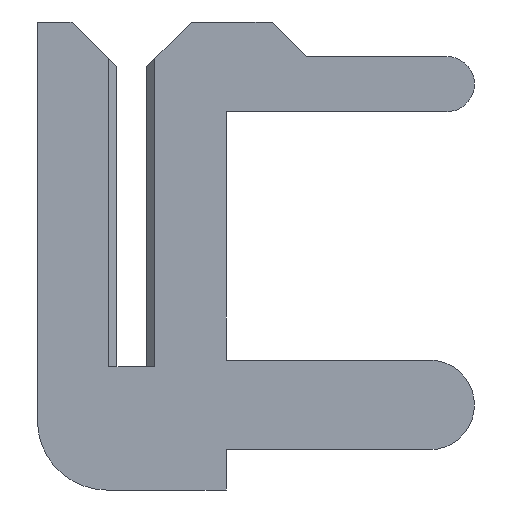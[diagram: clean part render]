
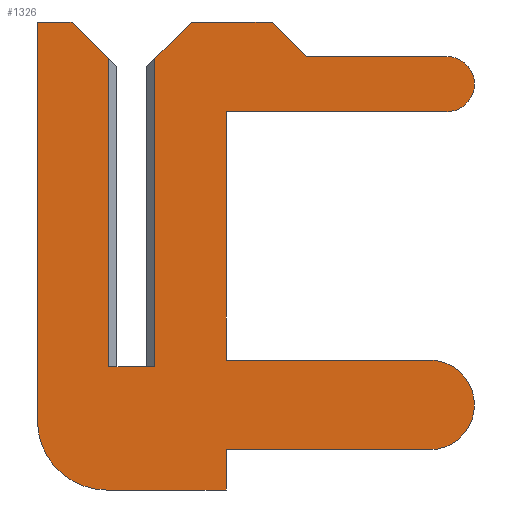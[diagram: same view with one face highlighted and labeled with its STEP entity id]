
A CAD part, left-side view. The second image highlights one B-rep face of the part: STEP entity #1326.
In plain terms, the highlighted planar face has unit normal (-1, 0, 0).
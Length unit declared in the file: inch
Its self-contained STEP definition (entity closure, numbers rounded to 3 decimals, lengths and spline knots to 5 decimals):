
#25 = VECTOR ( 'NONE', #924, 39.37008 ) ;
#30 = EDGE_CURVE ( 'NONE', #459, #676, #1230, .T. ) ;
#34 = CARTESIAN_POINT ( 'NONE',  ( -0.01, -0.041, -0.036 ) ) ;
#63 = DIRECTION ( 'NONE',  ( 0., 0., 1. ) ) ;
#75 = LINE ( 'NONE', #409, #1272 ) ;
#92 = CARTESIAN_POINT ( 'NONE',  ( -0.01, -0.041, -0.036 ) ) ;
#99 = ORIENTED_EDGE ( 'NONE', *, *, #148, .F. ) ;
#102 = CARTESIAN_POINT ( 'NONE',  ( -0.01, -0.1295, 0.003 ) ) ;
#108 = CIRCLE ( 'NONE', #139, 0.0195 ) ;
#113 = CARTESIAN_POINT ( 'NONE',  ( -0.01, -0.026, 0.15 ) ) ;
#116 = DIRECTION ( 'NONE',  ( 1., 0., 0. ) ) ;
#126 = VECTOR ( 'NONE', #713, 39.37008 ) ;
#127 = EDGE_CURVE ( 'NONE', #171, #828, #289, .T. ) ;
#139 = AXIS2_PLACEMENT_3D ( 'NONE', #839, #142, #849 ) ;
#142 = DIRECTION ( 'NONE',  ( 1., 0., 0. ) ) ;
#148 = EDGE_CURVE ( 'NONE', #936, #709, #663, .T. ) ;
#159 = VERTEX_POINT ( 'NONE', #92 ) ;
#171 = VERTEX_POINT ( 'NONE', #187 ) ;
#174 = DIRECTION ( 'NONE',  ( 1., 0., 0. ) ) ;
#179 = ORIENTED_EDGE ( 'NONE', *, *, #30, .F. ) ;
#186 = VECTOR ( 'NONE', #391, 39.37008 ) ;
#187 = CARTESIAN_POINT ( 'NONE',  ( -0.01, -0.041, -0.0535 ) ) ;
#191 = LINE ( 'NONE', #812, #1374 ) ;
#193 = ORIENTED_EDGE ( 'NONE', *, *, #1288, .F. ) ;
#198 = CARTESIAN_POINT ( 'NONE',  ( -0.01, -0.076, 0.135 ) ) ;
#202 = ORIENTED_EDGE ( 'NONE', *, *, #1087, .F. ) ;
#218 = ORIENTED_EDGE ( 'NONE', *, *, #1364, .F. ) ;
#219 = EDGE_CURVE ( 'NONE', #491, #324, #75, .T. ) ;
#234 = CARTESIAN_POINT ( 'NONE',  ( -0.01, -0.041, -0.0535 ) ) ;
#242 = DIRECTION ( 'NONE',  ( 0., 0., -1. ) ) ;
#253 = CARTESIAN_POINT ( 'NONE',  ( -0.01, -0.01, 0.134 ) ) ;
#268 = CARTESIAN_POINT ( 'NONE',  ( -0.01, -0.1295, 0.003 ) ) ;
#270 = VECTOR ( 'NONE', #474, 39.37008 ) ;
#289 = LINE ( 'NONE', #637, #1474 ) ;
#307 = ORIENTED_EDGE ( 'NONE', *, *, #879, .T. ) ;
#310 = LINE ( 'NONE', #342, #270 ) ;
#312 = VECTOR ( 'NONE', #1359, 39.37008 ) ;
#324 = VERTEX_POINT ( 'NONE', #526 ) ;
#336 = LINE ( 'NONE', #1060, #126 ) ;
#341 = EDGE_CURVE ( 'NONE', #1260, #595, #807, .T. ) ;
#342 = CARTESIAN_POINT ( 'NONE',  ( -0.01, 0.0065, 0. ) ) ;
#359 = DIRECTION ( 'NONE',  ( 0., 0., -1. ) ) ;
#373 = VECTOR ( 'NONE', #1048, 39.37008 ) ;
#380 = CARTESIAN_POINT ( 'NONE',  ( -0.01, 0.011, -0.0535 ) ) ;
#384 = CARTESIAN_POINT ( 'NONE',  ( -0.01, 0.011, -0.0235 ) ) ;
#391 = DIRECTION ( 'NONE',  ( 0., -1., 0. ) ) ;
#409 = CARTESIAN_POINT ( 'NONE',  ( -0.01, 0.0065, 0.1305 ) ) ;
#458 = CARTESIAN_POINT ( 'NONE',  ( -0.01, -0.137, 0.135 ) ) ;
#459 = VERTEX_POINT ( 'NONE', #1263 ) ;
#471 = ORIENTED_EDGE ( 'NONE', *, *, #1324, .F. ) ;
#473 = EDGE_CURVE ( 'NONE', #1168, #1331, #310, .T. ) ;
#474 = DIRECTION ( 'NONE',  ( 0., -1., 0. ) ) ;
#479 = CARTESIAN_POINT ( 'NONE',  ( -0.01, -0.0065, 0.1305 ) ) ;
#482 = CARTESIAN_POINT ( 'NONE',  ( -0.01, -0.026, 0.15 ) ) ;
#485 = LINE ( 'NONE', #234, #684 ) ;
#491 = VERTEX_POINT ( 'NONE', #926 ) ;
#496 = ORIENTED_EDGE ( 'NONE', *, *, #127, .F. ) ;
#505 = LINE ( 'NONE', #268, #186 ) ;
#517 = AXIS2_PLACEMENT_3D ( 'NONE', #384, #116, #825 ) ;
#526 = CARTESIAN_POINT ( 'NONE',  ( -0.01, 0.01, 0.134 ) ) ;
#531 = DIRECTION ( 'NONE',  ( 0., 1., 0. ) ) ;
#539 = VERTEX_POINT ( 'NONE', #458 ) ;
#562 = AXIS2_PLACEMENT_3D ( 'NONE', #1453, #174, #1429 ) ;
#595 = VERTEX_POINT ( 'NONE', #1037 ) ;
#597 = DIRECTION ( 'NONE',  ( 0., 0., 1. ) ) ;
#628 = LINE ( 'NONE', #1163, #870 ) ;
#637 = CARTESIAN_POINT ( 'NONE',  ( -0.01, 0.011, -0.0535 ) ) ;
#641 = VERTEX_POINT ( 'NONE', #102 ) ;
#647 = LINE ( 'NONE', #738, #702 ) ;
#660 = VECTOR ( 'NONE', #63, 39.37008 ) ;
#663 = LINE ( 'NONE', #1104, #312 ) ;
#676 = VERTEX_POINT ( 'NONE', #1307 ) ;
#684 = VECTOR ( 'NONE', #242, 39.37008 ) ;
#686 = EDGE_CURVE ( 'NONE', #828, #1260, #834, .T. ) ;
#687 = ORIENTED_EDGE ( 'NONE', *, *, #686, .F. ) ;
#698 = DIRECTION ( 'NONE',  ( 0., 1., 0. ) ) ;
#702 = VECTOR ( 'NONE', #880, 39.37008 ) ;
#707 = ORIENTED_EDGE ( 'NONE', *, *, #1242, .F. ) ;
#709 = VERTEX_POINT ( 'NONE', #1166 ) ;
#713 = DIRECTION ( 'NONE',  ( 0., 1., 0. ) ) ;
#715 = ORIENTED_EDGE ( 'NONE', *, *, #473, .F. ) ;
#732 = CARTESIAN_POINT ( 'NONE',  ( -0.01, -0.01, 0. ) ) ;
#738 = CARTESIAN_POINT ( 'NONE',  ( -0.01, -0.137, 0.135 ) ) ;
#748 = VERTEX_POINT ( 'NONE', #482 ) ;
#774 = ORIENTED_EDGE ( 'NONE', *, *, #1169, .F. ) ;
#780 = VECTOR ( 'NONE', #1391, 39.37008 ) ;
#785 = ORIENTED_EDGE ( 'NONE', *, *, #341, .F. ) ;
#807 = LINE ( 'NONE', #1325, #660 ) ;
#812 = CARTESIAN_POINT ( 'NONE',  ( -0.01, -0.01, 0.15 ) ) ;
#825 = DIRECTION ( 'NONE',  ( 0., 0., 1. ) ) ;
#828 = VERTEX_POINT ( 'NONE', #380 ) ;
#831 = VECTOR ( 'NONE', #698, 39.37008 ) ;
#834 = CIRCLE ( 'NONE', #517, 0.03 ) ;
#839 = CARTESIAN_POINT ( 'NONE',  ( -0.01, -0.1295, -0.0165 ) ) ;
#849 = DIRECTION ( 'NONE',  ( 0., 0., 1. ) ) ;
#870 = VECTOR ( 'NONE', #597, 39.37008 ) ;
#879 = EDGE_CURVE ( 'NONE', #1224, #1331, #191, .T. ) ;
#880 = DIRECTION ( 'NONE',  ( 0., -1., 0. ) ) ;
#885 = EDGE_LOOP ( 'NONE', ( #1437, #307, #715, #1167, #1149, #202, #785, #687, #496, #774, #1412, #193, #471, #99, #218, #1154, #1150, #179, #707 ) ) ;
#924 = DIRECTION ( 'NONE',  ( 0., -1., 0. ) ) ;
#926 = CARTESIAN_POINT ( 'NONE',  ( -0.01, 0.026, 0.15 ) ) ;
#931 = CARTESIAN_POINT ( 'NONE',  ( -0.01, 0.01, 0. ) ) ;
#936 = VERTEX_POINT ( 'NONE', #1202 ) ;
#944 = LINE ( 'NONE', #34, #831 ) ;
#958 = PLANE ( 'NONE',  #1228 ) ;
#992 = FACE_OUTER_BOUND ( 'NONE', #885, .T. ) ;
#1008 = EDGE_CURVE ( 'NONE', #1361, #159, #944, .T. ) ;
#1037 = CARTESIAN_POINT ( 'NONE',  ( -0.01, 0.041, 0.15 ) ) ;
#1048 = DIRECTION ( 'NONE',  ( 0., -0.707, 0.707 ) ) ;
#1060 = CARTESIAN_POINT ( 'NONE',  ( -0.01, -0.041, 0.111 ) ) ;
#1069 = LINE ( 'NONE', #113, #25 ) ;
#1087 = EDGE_CURVE ( 'NONE', #595, #491, #1329, .T. ) ;
#1104 = CARTESIAN_POINT ( 'NONE',  ( -0.01, -0.041, 0.003 ) ) ;
#1107 = LINE ( 'NONE', #479, #373 ) ;
#1111 = EDGE_CURVE ( 'NONE', #1168, #324, #628, .T. ) ;
#1123 = DIRECTION ( 'NONE',  ( 0., -0.707, -0.707 ) ) ;
#1149 = ORIENTED_EDGE ( 'NONE', *, *, #219, .F. ) ;
#1150 = ORIENTED_EDGE ( 'NONE', *, *, #1456, .F. ) ;
#1154 = ORIENTED_EDGE ( 'NONE', *, *, #1400, .F. ) ;
#1156 = CARTESIAN_POINT ( 'NONE',  ( -0.01, 0.041, -0.0235 ) ) ;
#1163 = CARTESIAN_POINT ( 'NONE',  ( -0.01, 0.01, -0.0235 ) ) ;
#1166 = CARTESIAN_POINT ( 'NONE',  ( -0.01, -0.041, 0.003 ) ) ;
#1167 = ORIENTED_EDGE ( 'NONE', *, *, #1111, .T. ) ;
#1168 = VERTEX_POINT ( 'NONE', #931 ) ;
#1169 = EDGE_CURVE ( 'NONE', #159, #171, #485, .T. ) ;
#1170 = CARTESIAN_POINT ( 'NONE',  ( -0.01, 0.026, 0.15 ) ) ;
#1179 = CARTESIAN_POINT ( 'NONE',  ( -0.01, -0.1295, -0.036 ) ) ;
#1191 = EDGE_CURVE ( 'NONE', #1224, #748, #1107, .T. ) ;
#1202 = CARTESIAN_POINT ( 'NONE',  ( -0.01, -0.041, 0.111 ) ) ;
#1206 = DIRECTION ( 'NONE',  ( 0., -0.707, -0.707 ) ) ;
#1224 = VERTEX_POINT ( 'NONE', #253 ) ;
#1228 = AXIS2_PLACEMENT_3D ( 'NONE', #1314, #1320, #1411 ) ;
#1230 = LINE ( 'NONE', #198, #1380 ) ;
#1242 = EDGE_CURVE ( 'NONE', #748, #459, #1069, .T. ) ;
#1260 = VERTEX_POINT ( 'NONE', #1156 ) ;
#1263 = CARTESIAN_POINT ( 'NONE',  ( -0.01, -0.061, 0.15 ) ) ;
#1272 = VECTOR ( 'NONE', #1206, 39.37008 ) ;
#1288 = EDGE_CURVE ( 'NONE', #641, #1361, #108, .T. ) ;
#1307 = CARTESIAN_POINT ( 'NONE',  ( -0.01, -0.076, 0.135 ) ) ;
#1314 = CARTESIAN_POINT ( 'NONE',  ( -0.01, 0.011, -0.0235 ) ) ;
#1320 = DIRECTION ( 'NONE',  ( -1., 0., 0. ) ) ;
#1324 = EDGE_CURVE ( 'NONE', #709, #641, #505, .T. ) ;
#1325 = CARTESIAN_POINT ( 'NONE',  ( -0.01, 0.041, 0.15 ) ) ;
#1326 = ADVANCED_FACE ( 'NONE', ( #992 ), #958, .T. ) ;
#1329 = LINE ( 'NONE', #1170, #780 ) ;
#1331 = VERTEX_POINT ( 'NONE', #732 ) ;
#1359 = DIRECTION ( 'NONE',  ( 0., 0., -1. ) ) ;
#1361 = VERTEX_POINT ( 'NONE', #1179 ) ;
#1364 = EDGE_CURVE ( 'NONE', #1409, #936, #336, .T. ) ;
#1371 = CIRCLE ( 'NONE', #562, 0.012 ) ;
#1374 = VECTOR ( 'NONE', #359, 39.37008 ) ;
#1380 = VECTOR ( 'NONE', #1123, 39.37008 ) ;
#1391 = DIRECTION ( 'NONE',  ( 0., -1., 0. ) ) ;
#1400 = EDGE_CURVE ( 'NONE', #539, #1409, #1371, .T. ) ;
#1409 = VERTEX_POINT ( 'NONE', #1441 ) ;
#1411 = DIRECTION ( 'NONE',  ( 0., 0., 1. ) ) ;
#1412 = ORIENTED_EDGE ( 'NONE', *, *, #1008, .F. ) ;
#1429 = DIRECTION ( 'NONE',  ( 0., 0., 1. ) ) ;
#1437 = ORIENTED_EDGE ( 'NONE', *, *, #1191, .F. ) ;
#1441 = CARTESIAN_POINT ( 'NONE',  ( -0.01, -0.137, 0.111 ) ) ;
#1453 = CARTESIAN_POINT ( 'NONE',  ( -0.01, -0.137, 0.123 ) ) ;
#1456 = EDGE_CURVE ( 'NONE', #676, #539, #647, .T. ) ;
#1474 = VECTOR ( 'NONE', #531, 39.37008 ) ;
